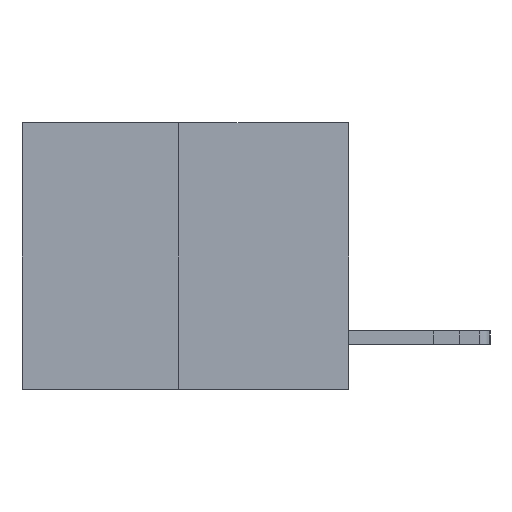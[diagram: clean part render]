
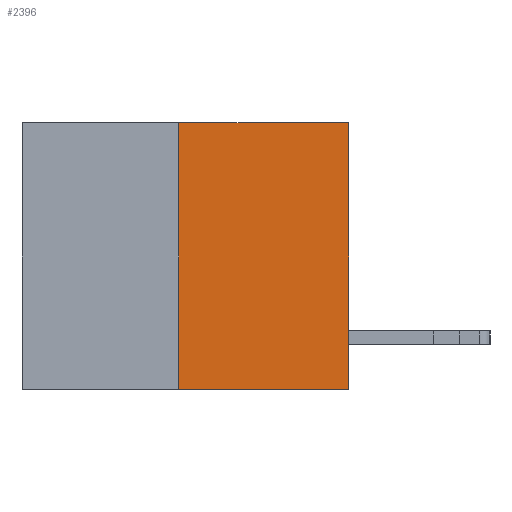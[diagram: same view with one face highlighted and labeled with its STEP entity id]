
A CAD part, left-side view. The second image highlights one B-rep face of the part: STEP entity #2396.
In plain terms, the highlighted planar face has unit normal (-1, 0, 0).
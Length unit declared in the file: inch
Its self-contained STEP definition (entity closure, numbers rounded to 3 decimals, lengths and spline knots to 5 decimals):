
#422 = EDGE_CURVE ( 'NONE', #5230, #9354, #3801, .T. ) ;
#474 = VECTOR ( 'NONE', #3121, 39.37008 ) ;
#936 = LINE ( 'NONE', #2981, #9095 ) ;
#1405 = VERTEX_POINT ( 'NONE', #13746 ) ;
#1634 = CARTESIAN_POINT ( 'NONE',  ( 0., 0.312, -0.49 ) ) ;
#1661 = LINE ( 'NONE', #10717, #474 ) ;
#1712 = CARTESIAN_POINT ( 'NONE',  ( 0., 0.6, -0.49 ) ) ;
#1761 = ORIENTED_EDGE ( 'NONE', *, *, #9821, .F. ) ;
#1963 = FACE_OUTER_BOUND ( 'NONE', #10374, .T. ) ;
#1982 = PLANE ( 'NONE',  #11611 ) ;
#2394 = VECTOR ( 'NONE', #2574, 39.37008 ) ;
#2396 = ADVANCED_FACE ( 'NONE', ( #1963 ), #1982, .F. ) ;
#2574 = DIRECTION ( 'NONE',  ( 0., -1., 0. ) ) ;
#2664 = VECTOR ( 'NONE', #12450, 39.37008 ) ;
#2981 = CARTESIAN_POINT ( 'NONE',  ( 0., 0., 0. ) ) ;
#3026 = CARTESIAN_POINT ( 'NONE',  ( 0., 0.6, 0. ) ) ;
#3121 = DIRECTION ( 'NONE',  ( 0., 0., 1. ) ) ;
#3801 = LINE ( 'NONE', #1712, #2664 ) ;
#4661 = CARTESIAN_POINT ( 'NONE',  ( 0., 0.6, 0. ) ) ;
#4857 = EDGE_CURVE ( 'NONE', #9354, #1405, #936, .T. ) ;
#5230 = VERTEX_POINT ( 'NONE', #1634 ) ;
#5584 = CARTESIAN_POINT ( 'NONE',  ( 0., 0., -0.49 ) ) ;
#6480 = EDGE_CURVE ( 'NONE', #9980, #1405, #10215, .T. ) ;
#6995 = ORIENTED_EDGE ( 'NONE', *, *, #4857, .T. ) ;
#9095 = VECTOR ( 'NONE', #9443, 39.37008 ) ;
#9354 = VERTEX_POINT ( 'NONE', #5584 ) ;
#9443 = DIRECTION ( 'NONE',  ( 0., 0., 1. ) ) ;
#9821 = EDGE_CURVE ( 'NONE', #5230, #9980, #1661, .T. ) ;
#9980 = VERTEX_POINT ( 'NONE', #11666 ) ;
#10215 = LINE ( 'NONE', #4661, #2394 ) ;
#10374 = EDGE_LOOP ( 'NONE', ( #1761, #12294, #6995, #11353 ) ) ;
#10498 = DIRECTION ( 'NONE',  ( 1., 0., 0. ) ) ;
#10717 = CARTESIAN_POINT ( 'NONE',  ( 0., 0.312, -0.49 ) ) ;
#11353 = ORIENTED_EDGE ( 'NONE', *, *, #6480, .F. ) ;
#11611 = AXIS2_PLACEMENT_3D ( 'NONE', #3026, #10498, #12681 ) ;
#11666 = CARTESIAN_POINT ( 'NONE',  ( 0., 0.312, 0. ) ) ;
#12294 = ORIENTED_EDGE ( 'NONE', *, *, #422, .T. ) ;
#12450 = DIRECTION ( 'NONE',  ( 0., -1., 0. ) ) ;
#12681 = DIRECTION ( 'NONE',  ( 0., 0., -1. ) ) ;
#13746 = CARTESIAN_POINT ( 'NONE',  ( 0., 0., 0. ) ) ;
